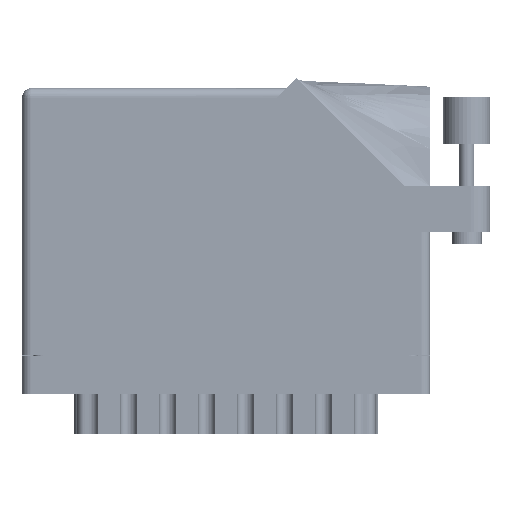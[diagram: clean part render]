
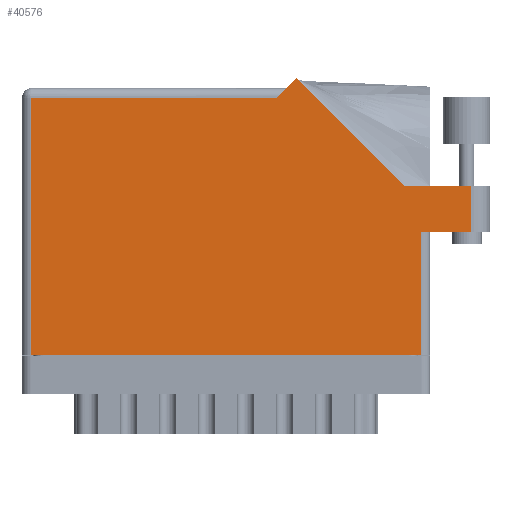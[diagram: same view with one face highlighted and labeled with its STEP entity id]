
A CAD part, front view. The second image highlights one B-rep face of the part: STEP entity #40576.
In plain terms, the highlighted face is planar.
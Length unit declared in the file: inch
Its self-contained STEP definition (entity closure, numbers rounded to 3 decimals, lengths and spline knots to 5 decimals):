
#116 = CARTESIAN_POINT ( 'NONE',  ( 2.656, 0.815, 0. ) ) ;
#1278 = EDGE_CURVE ( 'NONE', #20010, #46205, #28836, .T. ) ;
#2204 = ORIENTED_EDGE ( 'NONE', *, *, #14507, .T. ) ;
#4755 = ORIENTED_EDGE ( 'NONE', *, *, #61360, .T. ) ;
#7578 = DIRECTION ( 'NONE',  ( 1., 0., 0. ) ) ;
#8751 = CARTESIAN_POINT ( 'NONE',  ( 2.993, 0.815, 0. ) ) ;
#9327 = CARTESIAN_POINT ( 'NONE',  ( 2.993, 1.122, 0. ) ) ;
#9559 = VECTOR ( 'NONE', #7578, 39.37008 ) ;
#9579 = DIRECTION ( 'NONE',  ( 0., 1., 0. ) ) ;
#10211 = LINE ( 'NONE', #49405, #64952 ) ;
#11180 = LINE ( 'NONE', #75894, #13037 ) ;
#11648 = LINE ( 'NONE', #13164, #13502 ) ;
#12302 = CARTESIAN_POINT ( 'NONE',  ( 2.55242, 1.122, 0. ) ) ;
#13037 = VECTOR ( 'NONE', #17118, 39.37008 ) ;
#13164 = CARTESIAN_POINT ( 'NONE',  ( 1.758, 1.775, 0. ) ) ;
#13502 = VECTOR ( 'NONE', #24320, 39.37008 ) ;
#14507 = EDGE_CURVE ( 'NONE', #36444, #41977, #26181, .T. ) ;
#16851 = CARTESIAN_POINT ( 'NONE',  ( 1.82871, 1.84571, 0. ) ) ;
#17118 = DIRECTION ( 'NONE',  ( -1., 0., 0. ) ) ;
#17882 = CARTESIAN_POINT ( 'NONE',  ( 1.696, 1.713, 0. ) ) ;
#20010 = VERTEX_POINT ( 'NONE', #32885 ) ;
#20541 = CARTESIAN_POINT ( 'NONE',  ( 0., 0., 0. ) ) ;
#20564 = VECTOR ( 'NONE', #70292, 39.37008 ) ;
#22087 = LINE ( 'NONE', #56807, #44300 ) ;
#24320 = DIRECTION ( 'NONE',  ( -0.707, -0.707, 0. ) ) ;
#26072 = CARTESIAN_POINT ( 'NONE',  ( 2.656, 0., 0. ) ) ;
#26181 = LINE ( 'NONE', #116, #20564 ) ;
#26376 = ORIENTED_EDGE ( 'NONE', *, *, #54701, .T. ) ;
#26865 = CARTESIAN_POINT ( 'NONE',  ( 2.55242, 1.122, 0. ) ) ;
#28314 = ORIENTED_EDGE ( 'NONE', *, *, #37650, .T. ) ;
#28836 = LINE ( 'NONE', #49649, #72389 ) ;
#28903 = CARTESIAN_POINT ( 'NONE',  ( 2.656, 0.815, 0. ) ) ;
#30518 = ORIENTED_EDGE ( 'NONE', *, *, #72619, .T. ) ;
#32111 = AXIS2_PLACEMENT_3D ( 'NONE', #56213, #44774, #45275 ) ;
#32735 = DIRECTION ( 'NONE',  ( 1., 0., 0. ) ) ;
#32885 = CARTESIAN_POINT ( 'NONE',  ( 2.993, 1.122, 0. ) ) ;
#35220 = VERTEX_POINT ( 'NONE', #16851 ) ;
#35530 = LINE ( 'NONE', #20541, #9559 ) ;
#35785 = LINE ( 'NONE', #12302, #36665 ) ;
#36444 = VERTEX_POINT ( 'NONE', #26072 ) ;
#36665 = VECTOR ( 'NONE', #41294, 39.37008 ) ;
#37650 = EDGE_CURVE ( 'NONE', #50716, #55244, #10211, .T. ) ;
#40576 = ADVANCED_FACE ( 'NONE', ( #49467 ), #55961, .F. ) ;
#41294 = DIRECTION ( 'NONE',  ( -0.707, 0.707, 0. ) ) ;
#41977 = VERTEX_POINT ( 'NONE', #28903 ) ;
#43302 = EDGE_LOOP ( 'NONE', ( #53913, #30518, #52721, #50814, #66904, #4755, #28314, #26376, #2204 ) ) ;
#43303 = EDGE_CURVE ( 'NONE', #35220, #65357, #11648, .T. ) ;
#43445 = DIRECTION ( 'NONE',  ( 0., -1., 0. ) ) ;
#44300 = VECTOR ( 'NONE', #32735, 39.37008 ) ;
#44774 = DIRECTION ( 'NONE',  ( 0., 0., -1. ) ) ;
#45275 = DIRECTION ( 'NONE',  ( -1., 0., 0. ) ) ;
#45670 = LINE ( 'NONE', #9327, #58694 ) ;
#46205 = VERTEX_POINT ( 'NONE', #26865 ) ;
#49405 = CARTESIAN_POINT ( 'NONE',  ( 0.062, 0., 0. ) ) ;
#49467 = FACE_OUTER_BOUND ( 'NONE', #43302, .T. ) ;
#49649 = CARTESIAN_POINT ( 'NONE',  ( 3.118, 1.122, 0. ) ) ;
#50716 = VERTEX_POINT ( 'NONE', #64849 ) ;
#50814 = ORIENTED_EDGE ( 'NONE', *, *, #58240, .T. ) ;
#51428 = DIRECTION ( 'NONE',  ( -1., 0., 0. ) ) ;
#52721 = ORIENTED_EDGE ( 'NONE', *, *, #1278, .T. ) ;
#53913 = ORIENTED_EDGE ( 'NONE', *, *, #68890, .T. ) ;
#54701 = EDGE_CURVE ( 'NONE', #55244, #36444, #35530, .T. ) ;
#55244 = VERTEX_POINT ( 'NONE', #60381 ) ;
#55961 = PLANE ( 'NONE',  #32111 ) ;
#56213 = CARTESIAN_POINT ( 'NONE',  ( 0., 1.775, 0. ) ) ;
#56807 = CARTESIAN_POINT ( 'NONE',  ( 2.718, 0.815, 0. ) ) ;
#58240 = EDGE_CURVE ( 'NONE', #46205, #35220, #35785, .T. ) ;
#58694 = VECTOR ( 'NONE', #9579, 39.37008 ) ;
#60381 = CARTESIAN_POINT ( 'NONE',  ( 0.062, 0., 0. ) ) ;
#61360 = EDGE_CURVE ( 'NONE', #65357, #50716, #11180, .T. ) ;
#64849 = CARTESIAN_POINT ( 'NONE',  ( 0.062, 1.713, 0. ) ) ;
#64952 = VECTOR ( 'NONE', #43445, 39.37008 ) ;
#65357 = VERTEX_POINT ( 'NONE', #17882 ) ;
#66904 = ORIENTED_EDGE ( 'NONE', *, *, #43303, .T. ) ;
#68890 = EDGE_CURVE ( 'NONE', #41977, #74390, #22087, .T. ) ;
#70292 = DIRECTION ( 'NONE',  ( 0., 1., 0. ) ) ;
#72389 = VECTOR ( 'NONE', #51428, 39.37008 ) ;
#72619 = EDGE_CURVE ( 'NONE', #74390, #20010, #45670, .T. ) ;
#74390 = VERTEX_POINT ( 'NONE', #8751 ) ;
#75894 = CARTESIAN_POINT ( 'NONE',  ( 0., 1.713, 0. ) ) ;
